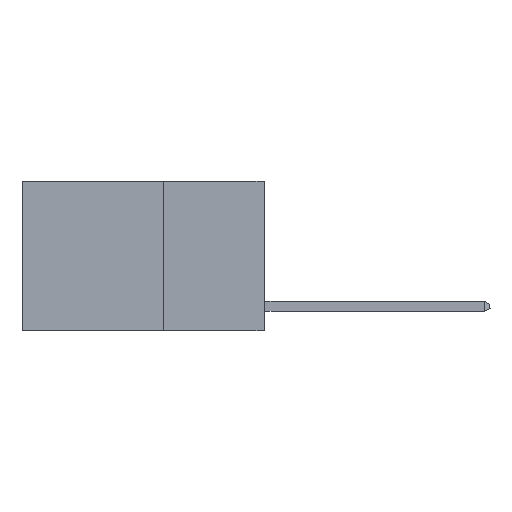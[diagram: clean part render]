
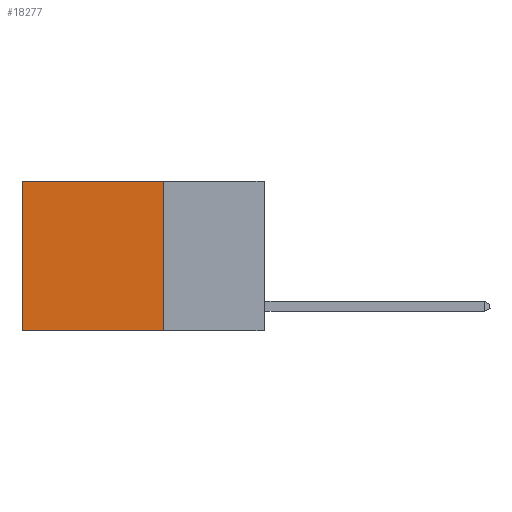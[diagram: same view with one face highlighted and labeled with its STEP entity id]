
A CAD part, left-side view. The second image highlights one B-rep face of the part: STEP entity #18277.
In plain terms, the highlighted planar face has unit normal (-1, 0, 0).
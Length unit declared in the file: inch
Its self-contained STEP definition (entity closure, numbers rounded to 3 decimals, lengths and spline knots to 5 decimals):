
#414 = ORIENTED_EDGE ( 'NONE', *, *, #12818, .F. ) ;
#1459 = EDGE_LOOP ( 'NONE', ( #6827, #20153, #414, #1888 ) ) ;
#1673 = VERTEX_POINT ( 'NONE', #17657 ) ;
#1872 = PLANE ( 'NONE',  #5114 ) ;
#1876 = VECTOR ( 'NONE', #3743, 39.37008 ) ;
#1888 = ORIENTED_EDGE ( 'NONE', *, *, #6083, .T. ) ;
#3743 = DIRECTION ( 'NONE',  ( 0., 0., -1. ) ) ;
#4211 = EDGE_CURVE ( 'NONE', #9522, #1673, #5803, .T. ) ;
#5114 = AXIS2_PLACEMENT_3D ( 'NONE', #17173, #6681, #13936 ) ;
#5150 = LINE ( 'NONE', #11446, #12141 ) ;
#5508 = CARTESIAN_POINT ( 'NONE',  ( 0.2625, 0.25, 0. ) ) ;
#5700 = VERTEX_POINT ( 'NONE', #11375 ) ;
#5803 = LINE ( 'NONE', #13866, #10321 ) ;
#6083 = EDGE_CURVE ( 'NONE', #5700, #9522, #19488, .T. ) ;
#6681 = DIRECTION ( 'NONE',  ( 1., 0., 0. ) ) ;
#6827 = ORIENTED_EDGE ( 'NONE', *, *, #4211, .T. ) ;
#6927 = VERTEX_POINT ( 'NONE', #20493 ) ;
#7013 = VECTOR ( 'NONE', #9851, 39.37008 ) ;
#7200 = LINE ( 'NONE', #5508, #1876 ) ;
#9522 = VERTEX_POINT ( 'NONE', #17563 ) ;
#9851 = DIRECTION ( 'NONE',  ( 0., 1., 0. ) ) ;
#10321 = VECTOR ( 'NONE', #20259, 39.37008 ) ;
#11375 = CARTESIAN_POINT ( 'NONE',  ( 0.2625, 0.25, 0. ) ) ;
#11446 = CARTESIAN_POINT ( 'NONE',  ( 0.2625, 0.25, -0.37 ) ) ;
#12141 = VECTOR ( 'NONE', #17926, 39.37008 ) ;
#12818 = EDGE_CURVE ( 'NONE', #5700, #6927, #7200, .T. ) ;
#13866 = CARTESIAN_POINT ( 'NONE',  ( 0.2625, 0.6, 0. ) ) ;
#13936 = DIRECTION ( 'NONE',  ( 0., 0., -1. ) ) ;
#15694 = FACE_OUTER_BOUND ( 'NONE', #1459, .T. ) ;
#17173 = CARTESIAN_POINT ( 'NONE',  ( 0.2625, 0.25, 0. ) ) ;
#17563 = CARTESIAN_POINT ( 'NONE',  ( 0.2625, 0.6, 0. ) ) ;
#17657 = CARTESIAN_POINT ( 'NONE',  ( 0.2625, 0.6, -0.37 ) ) ;
#17907 = CARTESIAN_POINT ( 'NONE',  ( 0.2625, 0.25, 0. ) ) ;
#17926 = DIRECTION ( 'NONE',  ( 0., 1., 0. ) ) ;
#18043 = EDGE_CURVE ( 'NONE', #6927, #1673, #5150, .T. ) ;
#18277 = ADVANCED_FACE ( 'NONE', ( #15694 ), #1872, .F. ) ;
#19488 = LINE ( 'NONE', #17907, #7013 ) ;
#20153 = ORIENTED_EDGE ( 'NONE', *, *, #18043, .F. ) ;
#20259 = DIRECTION ( 'NONE',  ( 0., 0., -1. ) ) ;
#20493 = CARTESIAN_POINT ( 'NONE',  ( 0.2625, 0.25, -0.37 ) ) ;
